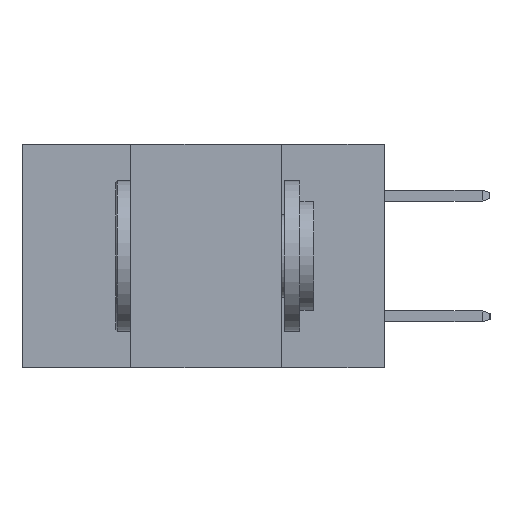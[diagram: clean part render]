
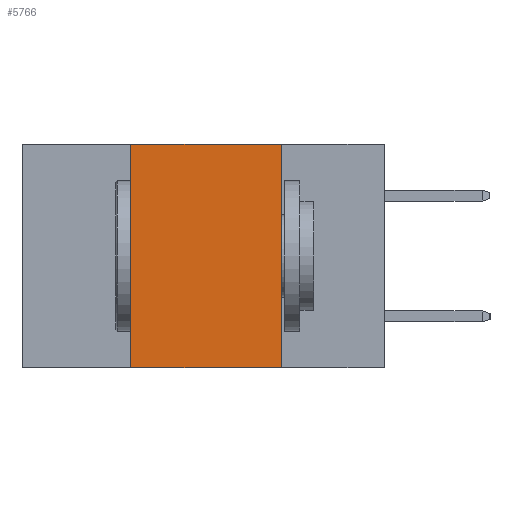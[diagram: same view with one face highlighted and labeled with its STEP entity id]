
A CAD part, left-side view. The second image highlights one B-rep face of the part: STEP entity #5766.
In plain terms, the highlighted planar face has unit normal (-1, 0, 0).
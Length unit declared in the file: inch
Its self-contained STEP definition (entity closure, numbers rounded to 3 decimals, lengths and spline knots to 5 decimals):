
#262 = FACE_OUTER_BOUND ( 'NONE', #5565, .T. ) ;
#801 = EDGE_CURVE ( 'NONE', #12213, #12574, #14660, .T. ) ;
#2054 = CARTESIAN_POINT ( 'NONE',  ( 0., 0.17, 0. ) ) ;
#2391 = VECTOR ( 'NONE', #4059, 39.37008 ) ;
#2555 = VERTEX_POINT ( 'NONE', #10600 ) ;
#2861 = VECTOR ( 'NONE', #10026, 39.37008 ) ;
#2914 = EDGE_CURVE ( 'NONE', #2555, #5977, #17291, .T. ) ;
#4057 = ORIENTED_EDGE ( 'NONE', *, *, #801, .T. ) ;
#4059 = DIRECTION ( 'NONE',  ( 0., 0., 1. ) ) ;
#5414 = DIRECTION ( 'NONE',  ( 0., 0., -1. ) ) ;
#5477 = DIRECTION ( 'NONE',  ( 1., 0., 0. ) ) ;
#5565 = EDGE_LOOP ( 'NONE', ( #17217, #17618, #10898, #4057 ) ) ;
#5567 = PLANE ( 'NONE',  #13790 ) ;
#5766 = ADVANCED_FACE ( 'NONE', ( #262 ), #5567, .F. ) ;
#5977 = VERTEX_POINT ( 'NONE', #2054 ) ;
#6204 = CARTESIAN_POINT ( 'NONE',  ( 0., 0.6, 0. ) ) ;
#6233 = CARTESIAN_POINT ( 'NONE',  ( 0., 0.42, -0.37 ) ) ;
#6448 = LINE ( 'NONE', #13613, #2391 ) ;
#6779 = VECTOR ( 'NONE', #9283, 39.37008 ) ;
#6822 = CARTESIAN_POINT ( 'NONE',  ( 0., 0.17, -0.37 ) ) ;
#6952 = VECTOR ( 'NONE', #10510, 39.37008 ) ;
#8141 = EDGE_CURVE ( 'NONE', #12213, #2555, #6448, .T. ) ;
#9283 = DIRECTION ( 'NONE',  ( 0., 0., -1. ) ) ;
#10026 = DIRECTION ( 'NONE',  ( 0., -1., 0. ) ) ;
#10510 = DIRECTION ( 'NONE',  ( 0., -1., 0. ) ) ;
#10600 = CARTESIAN_POINT ( 'NONE',  ( 0., 0.42, 0. ) ) ;
#10857 = LINE ( 'NONE', #6822, #6779 ) ;
#10898 = ORIENTED_EDGE ( 'NONE', *, *, #8141, .F. ) ;
#11003 = CARTESIAN_POINT ( 'NONE',  ( 0., 0.17, -0.37 ) ) ;
#11350 = CARTESIAN_POINT ( 'NONE',  ( 0., 0.6, 0. ) ) ;
#12213 = VERTEX_POINT ( 'NONE', #6233 ) ;
#12574 = VERTEX_POINT ( 'NONE', #11003 ) ;
#13613 = CARTESIAN_POINT ( 'NONE',  ( 0., 0.42, -0.37 ) ) ;
#13790 = AXIS2_PLACEMENT_3D ( 'NONE', #6204, #5477, #5414 ) ;
#14660 = LINE ( 'NONE', #17398, #6952 ) ;
#14706 = EDGE_CURVE ( 'NONE', #5977, #12574, #10857, .T. ) ;
#17217 = ORIENTED_EDGE ( 'NONE', *, *, #14706, .F. ) ;
#17291 = LINE ( 'NONE', #11350, #2861 ) ;
#17398 = CARTESIAN_POINT ( 'NONE',  ( 0., 0.6, -0.37 ) ) ;
#17618 = ORIENTED_EDGE ( 'NONE', *, *, #2914, .F. ) ;
